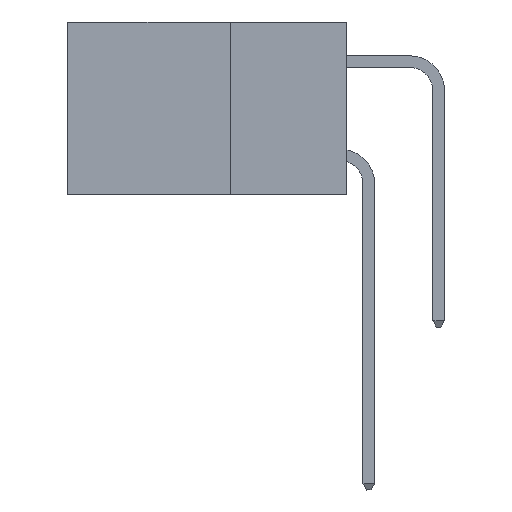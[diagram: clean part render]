
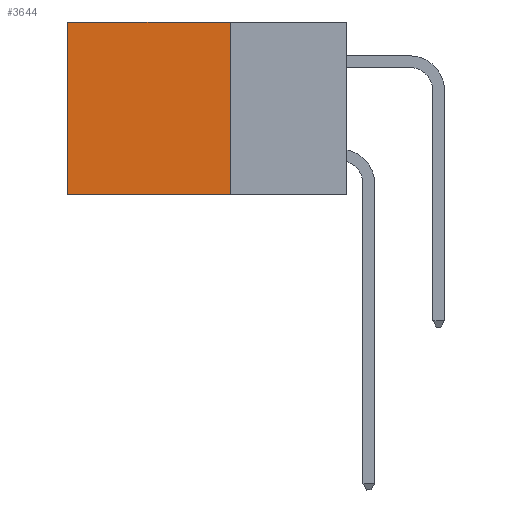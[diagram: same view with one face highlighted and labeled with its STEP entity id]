
A CAD part, left-side view. The second image highlights one B-rep face of the part: STEP entity #3644.
In plain terms, the highlighted planar face has unit normal (-1, 0, 0).
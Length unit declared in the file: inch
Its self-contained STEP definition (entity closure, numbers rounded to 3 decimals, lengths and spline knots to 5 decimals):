
#374 = FACE_OUTER_BOUND ( 'NONE', #16716, .T. ) ;
#733 = VERTEX_POINT ( 'NONE', #20270 ) ;
#765 = DIRECTION ( 'NONE',  ( 0., 1., 0. ) ) ;
#1043 = CARTESIAN_POINT ( 'NONE',  ( 0.2875, 0.6, -0.37 ) ) ;
#1581 = EDGE_CURVE ( 'NONE', #19213, #24221, #22976, .T. ) ;
#1834 = EDGE_CURVE ( 'NONE', #733, #24221, #18577, .T. ) ;
#2873 = PLANE ( 'NONE',  #21901 ) ;
#3479 = DIRECTION ( 'NONE',  ( 0., 0., -1. ) ) ;
#3644 = ADVANCED_FACE ( 'NONE', ( #374 ), #2873, .F. ) ;
#4044 = CARTESIAN_POINT ( 'NONE',  ( 0.2875, 0.25, 0. ) ) ;
#6117 = CARTESIAN_POINT ( 'NONE',  ( 0.2875, 0.6, 0. ) ) ;
#6688 = ORIENTED_EDGE ( 'NONE', *, *, #1834, .T. ) ;
#6792 = EDGE_CURVE ( 'NONE', #12100, #733, #14852, .T. ) ;
#7167 = DIRECTION ( 'NONE',  ( 0., 1., 0. ) ) ;
#8306 = CARTESIAN_POINT ( 'NONE',  ( 0.2875, 0.25, -0.37 ) ) ;
#8981 = VECTOR ( 'NONE', #765, 39.37008 ) ;
#9199 = CARTESIAN_POINT ( 'NONE',  ( 0.2875, 0.25, -0.37 ) ) ;
#10056 = DIRECTION ( 'NONE',  ( 0., 0., -1. ) ) ;
#12100 = VERTEX_POINT ( 'NONE', #4044 ) ;
#12295 = LINE ( 'NONE', #16585, #12565 ) ;
#12565 = VECTOR ( 'NONE', #3479, 39.37008 ) ;
#12882 = EDGE_CURVE ( 'NONE', #12100, #19213, #12295, .T. ) ;
#14852 = LINE ( 'NONE', #19667, #8981 ) ;
#15871 = ORIENTED_EDGE ( 'NONE', *, *, #12882, .F. ) ;
#16585 = CARTESIAN_POINT ( 'NONE',  ( 0.2875, 0.25, 0. ) ) ;
#16716 = EDGE_LOOP ( 'NONE', ( #6688, #23989, #15871, #23730 ) ) ;
#18335 = DIRECTION ( 'NONE',  ( 0., 0., -1. ) ) ;
#18577 = LINE ( 'NONE', #6117, #23842 ) ;
#19213 = VERTEX_POINT ( 'NONE', #8306 ) ;
#19667 = CARTESIAN_POINT ( 'NONE',  ( 0.2875, 0.25, 0. ) ) ;
#20270 = CARTESIAN_POINT ( 'NONE',  ( 0.2875, 0.6, 0. ) ) ;
#20283 = DIRECTION ( 'NONE',  ( 1., 0., 0. ) ) ;
#21527 = VECTOR ( 'NONE', #7167, 39.37008 ) ;
#21901 = AXIS2_PLACEMENT_3D ( 'NONE', #21980, #20283, #18335 ) ;
#21980 = CARTESIAN_POINT ( 'NONE',  ( 0.2875, 0.25, 0. ) ) ;
#22976 = LINE ( 'NONE', #9199, #21527 ) ;
#23730 = ORIENTED_EDGE ( 'NONE', *, *, #6792, .T. ) ;
#23842 = VECTOR ( 'NONE', #10056, 39.37008 ) ;
#23989 = ORIENTED_EDGE ( 'NONE', *, *, #1581, .F. ) ;
#24221 = VERTEX_POINT ( 'NONE', #1043 ) ;
